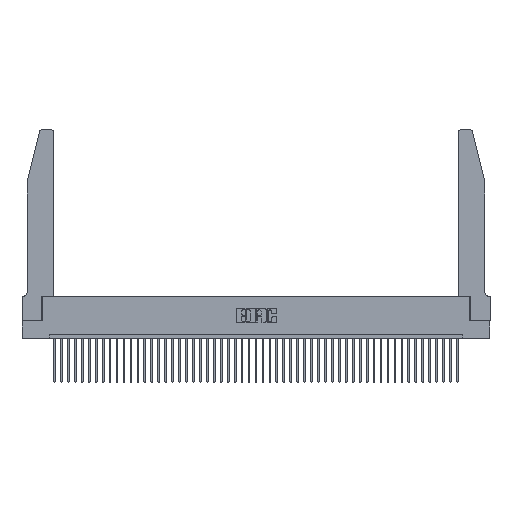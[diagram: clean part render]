
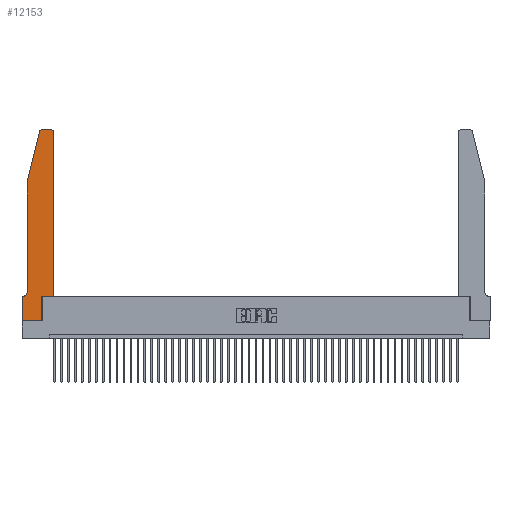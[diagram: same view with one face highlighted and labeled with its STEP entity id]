
A CAD part, top view. The second image highlights one B-rep face of the part: STEP entity #12153.
In plain terms, the highlighted planar face has unit normal (0, 0, 1).
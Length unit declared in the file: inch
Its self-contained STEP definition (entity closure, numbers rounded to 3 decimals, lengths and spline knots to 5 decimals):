
#294 = LINE ( 'NONE', #41752, #28609 ) ;
#631 = AXIS2_PLACEMENT_3D ( 'NONE', #16132, #1867, #12978 ) ;
#1011 = CIRCLE ( 'NONE', #44914, 0.03 ) ;
#1867 = DIRECTION ( 'NONE',  ( 0., 0., -1. ) ) ;
#2384 = DIRECTION ( 'NONE',  ( 0., 1., 0. ) ) ;
#2798 = LINE ( 'NONE', #21134, #14183 ) ;
#2971 = LINE ( 'NONE', #44753, #4651 ) ;
#3434 = CARTESIAN_POINT ( 'NONE',  ( 0.0755, 0.42, 0.37 ) ) ;
#4083 = EDGE_CURVE ( 'NONE', #14483, #10652, #28299, .T. ) ;
#4246 = LINE ( 'NONE', #33513, #18959 ) ;
#4419 = CARTESIAN_POINT ( 'NONE',  ( 0., 0., 0.37 ) ) ;
#4651 = VECTOR ( 'NONE', #26725, 39.37008 ) ;
#4916 = CARTESIAN_POINT ( 'NONE',  ( 0.0055, 0.35, 0.37 ) ) ;
#6500 = CARTESIAN_POINT ( 'NONE',  ( 0.4205, 2.75, 0.37 ) ) ;
#7143 = ORIENTED_EDGE ( 'NONE', *, *, #7909, .T. ) ;
#7557 = DIRECTION ( 'NONE',  ( 1., 0., 0. ) ) ;
#7909 = EDGE_CURVE ( 'NONE', #39101, #11437, #1011, .T. ) ;
#8018 = CARTESIAN_POINT ( 'NONE',  ( 0.284, 2.72, 0.37 ) ) ;
#8528 = EDGE_CURVE ( 'NONE', #42427, #13489, #43403, .T. ) ;
#8559 = ORIENTED_EDGE ( 'NONE', *, *, #27439, .T. ) ;
#9585 = ORIENTED_EDGE ( 'NONE', *, *, #27153, .T. ) ;
#10652 = VERTEX_POINT ( 'NONE', #3434 ) ;
#11243 = ORIENTED_EDGE ( 'NONE', *, *, #12222, .T. ) ;
#11364 = ORIENTED_EDGE ( 'NONE', *, *, #38870, .T. ) ;
#11437 = VERTEX_POINT ( 'NONE', #35728 ) ;
#11859 = DIRECTION ( 'NONE',  ( 0., 1., 0. ) ) ;
#12153 = ADVANCED_FACE ( 'NONE', ( #19305 ), #32534, .T. ) ;
#12222 = EDGE_CURVE ( 'NONE', #13489, #17155, #24415, .T. ) ;
#12978 = DIRECTION ( 'NONE',  ( -1., 0., 0. ) ) ;
#13475 = VECTOR ( 'NONE', #14622, 39.37008 ) ;
#13489 = VERTEX_POINT ( 'NONE', #32883 ) ;
#13612 = DIRECTION ( 'NONE',  ( 0., 0., 1. ) ) ;
#13764 = ORIENTED_EDGE ( 'NONE', *, *, #24077, .T. ) ;
#14183 = VECTOR ( 'NONE', #16879, 39.37008 ) ;
#14483 = VERTEX_POINT ( 'NONE', #30915 ) ;
#14563 = DIRECTION ( 'NONE',  ( 1., 0., 0. ) ) ;
#14622 = DIRECTION ( 'NONE',  ( 0., -1., 0. ) ) ;
#16132 = CARTESIAN_POINT ( 'NONE',  ( 0.0055, 0.42, 0.37 ) ) ;
#16498 = ORIENTED_EDGE ( 'NONE', *, *, #8528, .T. ) ;
#16879 = DIRECTION ( 'NONE',  ( -1., 0., 0. ) ) ;
#17155 = VERTEX_POINT ( 'NONE', #35275 ) ;
#17312 = DIRECTION ( 'NONE',  ( 1., 0., 0. ) ) ;
#17522 = CARTESIAN_POINT ( 'NONE',  ( 0.0755, 2., 0.37 ) ) ;
#17931 = ORIENTED_EDGE ( 'NONE', *, *, #26950, .T. ) ;
#18237 = CIRCLE ( 'NONE', #631, 0.07 ) ;
#18246 = VERTEX_POINT ( 'NONE', #6500 ) ;
#18302 = CARTESIAN_POINT ( 'NONE',  ( 0., 0., 0.37 ) ) ;
#18754 = DIRECTION ( 'NONE',  ( 1., 0., 0. ) ) ;
#18959 = VECTOR ( 'NONE', #11859, 39.37008 ) ;
#19305 = FACE_OUTER_BOUND ( 'NONE', #35812, .T. ) ;
#20938 = CARTESIAN_POINT ( 'NONE',  ( 0.2865, 0.35, 0.37 ) ) ;
#20999 = DIRECTION ( 'NONE',  ( 0., -1., 0. ) ) ;
#21134 = CARTESIAN_POINT ( 'NONE',  ( 0.0755, 0.35, 0.37 ) ) ;
#22104 = DIRECTION ( 'NONE',  ( 0., 0., 1. ) ) ;
#22178 = CARTESIAN_POINT ( 'NONE',  ( 0.4505, 0.35, 0.37 ) ) ;
#24063 = VERTEX_POINT ( 'NONE', #20938 ) ;
#24077 = EDGE_CURVE ( 'NONE', #29327, #18246, #43799, .T. ) ;
#24278 = DIRECTION ( 'NONE',  ( -0.239, -0.971, 0. ) ) ;
#24415 = LINE ( 'NONE', #18302, #39096 ) ;
#24740 = ORIENTED_EDGE ( 'NONE', *, *, #27918, .T. ) ;
#26725 = DIRECTION ( 'NONE',  ( -1., 0., 0. ) ) ;
#26887 = ORIENTED_EDGE ( 'NONE', *, *, #31337, .T. ) ;
#26950 = EDGE_CURVE ( 'NONE', #11437, #14483, #29797, .T. ) ;
#27153 = EDGE_CURVE ( 'NONE', #24063, #44599, #29196, .T. ) ;
#27439 = EDGE_CURVE ( 'NONE', #17155, #24063, #294, .T. ) ;
#27525 = VECTOR ( 'NONE', #24278, 39.37008 ) ;
#27918 = EDGE_CURVE ( 'NONE', #44599, #29327, #4246, .T. ) ;
#28065 = VECTOR ( 'NONE', #43840, 39.37008 ) ;
#28299 = LINE ( 'NONE', #17522, #38540 ) ;
#28609 = VECTOR ( 'NONE', #2384, 39.37008 ) ;
#29098 = EDGE_CURVE ( 'NONE', #10652, #41328, #18237, .T. ) ;
#29196 = LINE ( 'NONE', #22178, #28065 ) ;
#29327 = VERTEX_POINT ( 'NONE', #34291 ) ;
#29744 = ORIENTED_EDGE ( 'NONE', *, *, #29098, .T. ) ;
#29797 = LINE ( 'NONE', #35167, #27525 ) ;
#30915 = CARTESIAN_POINT ( 'NONE',  ( 0.0755, 2., 0.37 ) ) ;
#31337 = EDGE_CURVE ( 'NONE', #41328, #42427, #2798, .T. ) ;
#31440 = AXIS2_PLACEMENT_3D ( 'NONE', #42432, #35330, #17312 ) ;
#32534 = PLANE ( 'NONE',  #35385 ) ;
#32883 = CARTESIAN_POINT ( 'NONE',  ( 0., 0., 0.37 ) ) ;
#33513 = CARTESIAN_POINT ( 'NONE',  ( 0.4505, 0.35, 0.37 ) ) ;
#34291 = CARTESIAN_POINT ( 'NONE',  ( 0.4505, 2.72, 0.37 ) ) ;
#35167 = CARTESIAN_POINT ( 'NONE',  ( 0.0755, 2., 0.37 ) ) ;
#35275 = CARTESIAN_POINT ( 'NONE',  ( 0.2865, 0., 0.37 ) ) ;
#35330 = DIRECTION ( 'NONE',  ( 0., 0., 1. ) ) ;
#35385 = AXIS2_PLACEMENT_3D ( 'NONE', #36168, #13612, #14563 ) ;
#35728 = CARTESIAN_POINT ( 'NONE',  ( 0.25487, 2.72718, 0.37 ) ) ;
#35812 = EDGE_LOOP ( 'NONE', ( #11364, #7143, #17931, #40355, #29744, #26887, #16498, #11243, #8559, #9585, #24740, #13764 ) ) ;
#36168 = CARTESIAN_POINT ( 'NONE',  ( 0., 0.35, 0.37 ) ) ;
#38221 = CARTESIAN_POINT ( 'NONE',  ( 0., 0.35, 0.37 ) ) ;
#38540 = VECTOR ( 'NONE', #20999, 39.37008 ) ;
#38870 = EDGE_CURVE ( 'NONE', #18246, #39101, #2971, .T. ) ;
#39096 = VECTOR ( 'NONE', #18754, 39.37008 ) ;
#39101 = VERTEX_POINT ( 'NONE', #43314 ) ;
#39666 = CARTESIAN_POINT ( 'NONE',  ( 0.4505, 0.35, 0.37 ) ) ;
#40355 = ORIENTED_EDGE ( 'NONE', *, *, #4083, .T. ) ;
#41328 = VERTEX_POINT ( 'NONE', #4916 ) ;
#41752 = CARTESIAN_POINT ( 'NONE',  ( 0.2865, 0.35, 0.37 ) ) ;
#42427 = VERTEX_POINT ( 'NONE', #38221 ) ;
#42432 = CARTESIAN_POINT ( 'NONE',  ( 0.4205, 2.72, 0.37 ) ) ;
#43314 = CARTESIAN_POINT ( 'NONE',  ( 0.284, 2.75, 0.37 ) ) ;
#43403 = LINE ( 'NONE', #4419, #13475 ) ;
#43799 = CIRCLE ( 'NONE', #31440, 0.03 ) ;
#43840 = DIRECTION ( 'NONE',  ( 1., 0., 0. ) ) ;
#44599 = VERTEX_POINT ( 'NONE', #39666 ) ;
#44753 = CARTESIAN_POINT ( 'NONE',  ( 0.2605, 2.75, 0.37 ) ) ;
#44914 = AXIS2_PLACEMENT_3D ( 'NONE', #8018, #22104, #7557 ) ;
